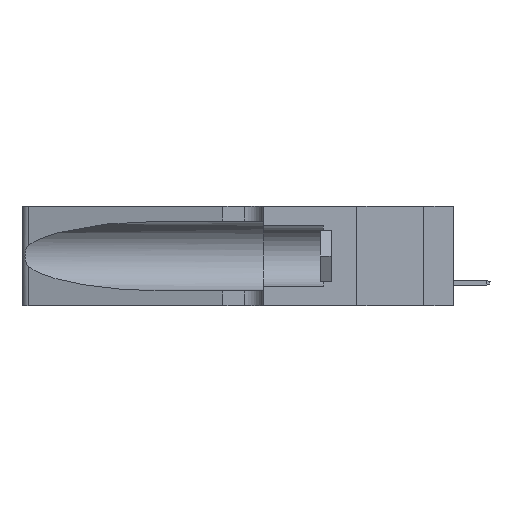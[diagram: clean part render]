
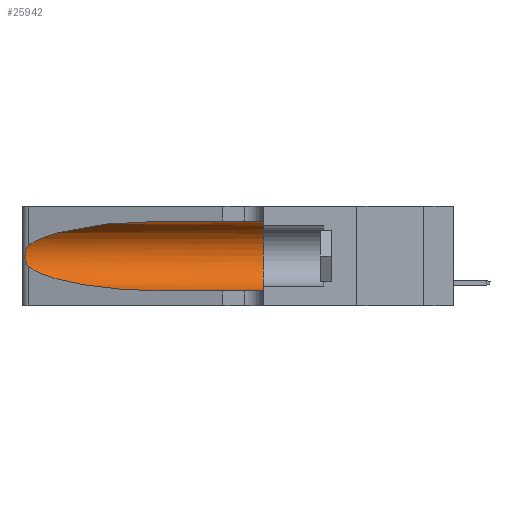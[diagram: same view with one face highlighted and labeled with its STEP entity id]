
A CAD part, left-side view. The second image highlights one B-rep face of the part: STEP entity #25942.
In plain terms, the highlighted cylindrical face has radius 3.308 mm (diameter 6.617 mm), a partial arc.
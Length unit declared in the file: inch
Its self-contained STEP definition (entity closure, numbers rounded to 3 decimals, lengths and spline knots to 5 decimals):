
#504 = VERTEX_POINT ( 'NONE', #17670 ) ;
#907 = EDGE_CURVE ( 'NONE', #23468, #504, #6358, .T. ) ;
#1209 = EDGE_CURVE ( 'NONE', #25380, #1889, #19603, .T. ) ;
#1889 = VERTEX_POINT ( 'NONE', #23255 ) ;
#2316 = VECTOR ( 'NONE', #6605, 39.37008 ) ;
#2862 = CARTESIAN_POINT ( 'NONE',  ( 0.25639, 1.23184, 0.21858 ) ) ;
#5234 = CARTESIAN_POINT ( 'NONE',  ( 0.25787, 1.23484, 0.2124 ) ) ;
#6142 = CARTESIAN_POINT ( 'NONE',  ( 0.25487, 1.22718, 0.14631 ) ) ;
#6160 = ORIENTED_EDGE ( 'NONE', *, *, #12779, .F. ) ;
#6217 = CARTESIAN_POINT ( 'NONE',  ( 0.1305, 0.35, 0.185 ) ) ;
#6358 = LINE ( 'NONE', #16646, #19539 ) ;
#6522 = DIRECTION ( 'NONE',  ( 0., -1., 0. ) ) ;
#6605 = DIRECTION ( 'NONE',  ( 0., -1., 0. ) ) ;
#7256 = CARTESIAN_POINT ( 'NONE',  ( 0.26075, 1.23896, 0.178 ) ) ;
#7622 = FACE_OUTER_BOUND ( 'NONE', #10963, .T. ) ;
#9962 = ORIENTED_EDGE ( 'NONE', *, *, #1209, .T. ) ;
#9968 = CARTESIAN_POINT ( 'NONE',  ( 0.25555, 1.22994, 0.2215 ) ) ;
#10322 = CARTESIAN_POINT ( 'NONE',  ( 0.1305, 0.72297, 0.05475 ) ) ;
#10445 = CARTESIAN_POINT ( 'NONE',  ( 0.25487, 1.22718, 0.22369 ) ) ;
#10963 = EDGE_LOOP ( 'NONE', ( #27586, #24969, #22798, #9962, #6160, #19049 ) ) ;
#12779 = EDGE_CURVE ( 'NONE', #504, #1889, #28095, .T. ) ;
#12833 = CARTESIAN_POINT ( 'NONE',  ( 0.26017, 1.23833, 0.17102 ) ) ;
#14474 = DIRECTION ( 'NONE',  ( 0., 0., 1. ) ) ;
#15525 = CARTESIAN_POINT ( 'NONE',  ( 0.25487, 1.22718, 0.22369 ) ) ;
#15904 = CARTESIAN_POINT ( 'NONE',  ( 0.1305, 0.72297, 0.31525 ) ) ;
#16646 = CARTESIAN_POINT ( 'NONE',  ( 0.1305, 1.61858, 0.31525 ) ) ;
#17354 = EDGE_CURVE ( 'NONE', #23468, #30681, #29520, .T. ) ;
#17558 = CARTESIAN_POINT ( 'NONE',  ( 0.25555, 1.22993, 0.14849 ) ) ;
#17599 = CARTESIAN_POINT ( 'NONE',  ( 0.1305, 1.61858, 0.185 ) ) ;
#17638 = CARTESIAN_POINT ( 'NONE',  ( 0.1305, 0.72297, 0.31525 ) ) ;
#17670 = CARTESIAN_POINT ( 'NONE',  ( 0.1305, 0.35, 0.31525 ) ) ;
#17920 = CYLINDRICAL_SURFACE ( 'NONE', #28133, 0.13025 ) ;
#18263 = DIRECTION ( 'NONE',  ( 0., 0., -1. ) ) ;
#19049 = ORIENTED_EDGE ( 'NONE', *, *, #907, .F. ) ;
#19539 = VECTOR ( 'NONE', #6522, 39.37008 ) ;
#19603 = LINE ( 'NONE', #29747, #2316 ) ;
#19839 = CARTESIAN_POINT ( 'NONE',  ( 0.2373, 1.15595, 0.28018 ) ) ;
#20174 = CARTESIAN_POINT ( 'NONE',  ( 0.25487, 1.22718, 0.22369 ) ) ;
#20258 = CARTESIAN_POINT ( 'NONE',  ( 0.26018, 1.23835, 0.19895 ) ) ;
#20417 = CARTESIAN_POINT ( 'NONE',  ( 0.25789, 1.23486, 0.15765 ) ) ;
#20450 = CARTESIAN_POINT ( 'NONE',  ( 0.25487, 1.22718, 0.14631 ) ) ;
#22050 = EDGE_CURVE ( 'NONE', #31722, #25380, #32951, .T. ) ;
#22547 = CARTESIAN_POINT ( 'NONE',  ( 0.18966, 0.96281, 0.31525 ) ) ;
#22629 = CARTESIAN_POINT ( 'NONE',  ( 0.26075, 1.23896, 0.19203 ) ) ;
#22798 = ORIENTED_EDGE ( 'NONE', *, *, #22050, .T. ) ;
#23002 = CARTESIAN_POINT ( 'NONE',  ( 0.2373, 1.15595, 0.08982 ) ) ;
#23223 = AXIS2_PLACEMENT_3D ( 'NONE', #6217, #29678, #14474 ) ;
#23255 = CARTESIAN_POINT ( 'NONE',  ( 0.1305, 0.35, 0.05475 ) ) ;
#23295 = CARTESIAN_POINT ( 'NONE',  ( 0.25487, 1.22718, 0.14631 ) ) ;
#23468 = VERTEX_POINT ( 'NONE', #15904 ) ;
#23873 = EDGE_CURVE ( 'NONE', #30681, #31722, #28354, .T. ) ;
#24969 = ORIENTED_EDGE ( 'NONE', *, *, #23873, .T. ) ;
#25251 = CARTESIAN_POINT ( 'NONE',  ( 0.1305, 0.72297, 0.05475 ) ) ;
#25380 = VERTEX_POINT ( 'NONE', #25251 ) ;
#25834 = CARTESIAN_POINT ( 'NONE',  ( 0.25639, 1.23186, 0.15144 ) ) ;
#25942 = ADVANCED_FACE ( 'NONE', ( #7622 ), #17920, .F. ) ;
#27586 = ORIENTED_EDGE ( 'NONE', *, *, #17354, .T. ) ;
#27909 = CARTESIAN_POINT ( 'NONE',  ( 0.18966, 0.96281, 0.05475 ) ) ;
#28095 = CIRCLE ( 'NONE', #23223, 0.13025 ) ;
#28133 = AXIS2_PLACEMENT_3D ( 'NONE', #17599, #28239, #18263 ) ;
#28239 = DIRECTION ( 'NONE',  ( 0., -1., 0. ) ) ;
#28354 = B_SPLINE_CURVE_WITH_KNOTS ( 'NONE', 3,
 ( #15525, #9968, #2862, #5234, #30397, #20258, #22629, #7256, #12833, #30566, #20417, #25834, #17558, #23295 ),
 .UNSPECIFIED., .F., .F.,
 ( 4, 2, 2, 2, 2, 2, 4 ),
 ( 0., 0.00027, 0.00053, 0.00107, 0.0016, 0.00187, 0.00214 ),
 .UNSPECIFIED. ) ;
#29520 =( BOUNDED_CURVE ( )  B_SPLINE_CURVE ( 3, ( #17638, #22547, #19839, #20174 ),
 .UNSPECIFIED., .F., .T. ) 
 B_SPLINE_CURVE_WITH_KNOTS ( ( 4, 4 ),
 ( 1.5708, 2.84003 ),
 .UNSPECIFIED. ) 
 CURVE ( )  GEOMETRIC_REPRESENTATION_ITEM ( )  RATIONAL_B_SPLINE_CURVE ( ( 1., 0.87, 0.87, 1. ) ) 
 REPRESENTATION_ITEM ( '' )  );
#29678 = DIRECTION ( 'NONE',  ( 0., 1., 0. ) ) ;
#29747 = CARTESIAN_POINT ( 'NONE',  ( 0.1305, 1.61858, 0.05475 ) ) ;
#30397 = CARTESIAN_POINT ( 'NONE',  ( 0.25854, 1.2359, 0.20912 ) ) ;
#30566 = CARTESIAN_POINT ( 'NONE',  ( 0.25856, 1.23593, 0.16098 ) ) ;
#30681 = VERTEX_POINT ( 'NONE', #10445 ) ;
#31722 = VERTEX_POINT ( 'NONE', #6142 ) ;
#32951 =( BOUNDED_CURVE ( )  B_SPLINE_CURVE ( 3, ( #20450, #23002, #27909, #10322 ),
 .UNSPECIFIED., .F., .T. ) 
 B_SPLINE_CURVE_WITH_KNOTS ( ( 4, 4 ),
 ( 3.44316, 4.71239 ),
 .UNSPECIFIED. ) 
 CURVE ( )  GEOMETRIC_REPRESENTATION_ITEM ( )  RATIONAL_B_SPLINE_CURVE ( ( 1., 0.87, 0.87, 1. ) ) 
 REPRESENTATION_ITEM ( '' )  );
